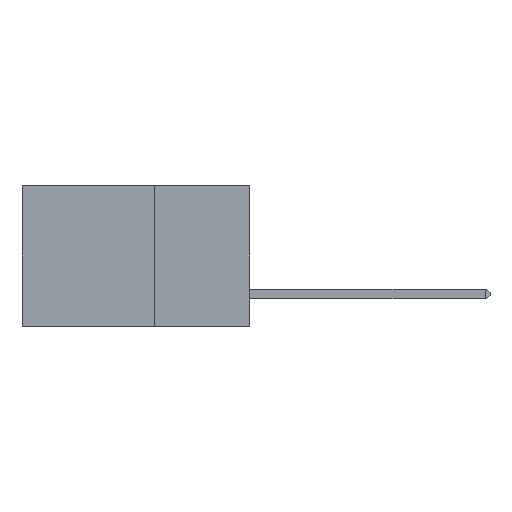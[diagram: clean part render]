
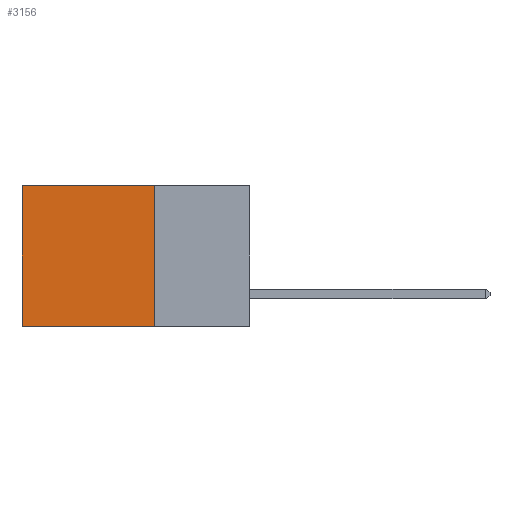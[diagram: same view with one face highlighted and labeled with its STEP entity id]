
A CAD part, left-side view. The second image highlights one B-rep face of the part: STEP entity #3156.
In plain terms, the highlighted planar face has unit normal (-1, 0, 0).
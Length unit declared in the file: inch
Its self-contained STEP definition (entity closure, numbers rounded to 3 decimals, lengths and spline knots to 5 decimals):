
#470 = ORIENTED_EDGE ( 'NONE', *, *, #1167, .F. ) ;
#757 = LINE ( 'NONE', #11314, #11843 ) ;
#1167 = EDGE_CURVE ( 'NONE', #13160, #4081, #2544, .T. ) ;
#1498 = CARTESIAN_POINT ( 'NONE',  ( 0.2875, 0.6, 0. ) ) ;
#2031 = CARTESIAN_POINT ( 'NONE',  ( 0.2875, 0.6, -0.37 ) ) ;
#2465 = VECTOR ( 'NONE', #11687, 39.37008 ) ;
#2514 = EDGE_CURVE ( 'NONE', #5695, #7132, #757, .T. ) ;
#2529 = ORIENTED_EDGE ( 'NONE', *, *, #2514, .T. ) ;
#2544 = LINE ( 'NONE', #4226, #11454 ) ;
#2608 = CARTESIAN_POINT ( 'NONE',  ( 0.2875, 0.25, -0.37 ) ) ;
#2815 = DIRECTION ( 'NONE',  ( 0., 0., -1. ) ) ;
#2835 = DIRECTION ( 'NONE',  ( 1., 0., 0. ) ) ;
#2887 = PLANE ( 'NONE',  #12755 ) ;
#3063 = CARTESIAN_POINT ( 'NONE',  ( 0.2875, 0.25, 0. ) ) ;
#3156 = ADVANCED_FACE ( 'NONE', ( #10305 ), #2887, .F. ) ;
#3536 = ORIENTED_EDGE ( 'NONE', *, *, #13777, .T. ) ;
#4081 = VERTEX_POINT ( 'NONE', #2031 ) ;
#4226 = CARTESIAN_POINT ( 'NONE',  ( 0.2875, 0.25, -0.37 ) ) ;
#4681 = VECTOR ( 'NONE', #7582, 39.37008 ) ;
#5695 = VERTEX_POINT ( 'NONE', #10103 ) ;
#6320 = EDGE_CURVE ( 'NONE', #5695, #13160, #14495, .T. ) ;
#6463 = DIRECTION ( 'NONE',  ( 0., 1., 0. ) ) ;
#7132 = VERTEX_POINT ( 'NONE', #1498 ) ;
#7371 = EDGE_LOOP ( 'NONE', ( #3536, #470, #7458, #2529 ) ) ;
#7458 = ORIENTED_EDGE ( 'NONE', *, *, #6320, .F. ) ;
#7582 = DIRECTION ( 'NONE',  ( 0., 0., -1. ) ) ;
#8186 = LINE ( 'NONE', #11994, #4681 ) ;
#9508 = CARTESIAN_POINT ( 'NONE',  ( 0.2875, 0.25, 0. ) ) ;
#10103 = CARTESIAN_POINT ( 'NONE',  ( 0.2875, 0.25, 0. ) ) ;
#10305 = FACE_OUTER_BOUND ( 'NONE', #7371, .T. ) ;
#11203 = DIRECTION ( 'NONE',  ( 0., 1., 0. ) ) ;
#11314 = CARTESIAN_POINT ( 'NONE',  ( 0.2875, 0.25, 0. ) ) ;
#11454 = VECTOR ( 'NONE', #6463, 39.37008 ) ;
#11687 = DIRECTION ( 'NONE',  ( 0., 0., -1. ) ) ;
#11843 = VECTOR ( 'NONE', #11203, 39.37008 ) ;
#11994 = CARTESIAN_POINT ( 'NONE',  ( 0.2875, 0.6, 0. ) ) ;
#12755 = AXIS2_PLACEMENT_3D ( 'NONE', #3063, #2835, #2815 ) ;
#13160 = VERTEX_POINT ( 'NONE', #2608 ) ;
#13777 = EDGE_CURVE ( 'NONE', #7132, #4081, #8186, .T. ) ;
#14495 = LINE ( 'NONE', #9508, #2465 ) ;
